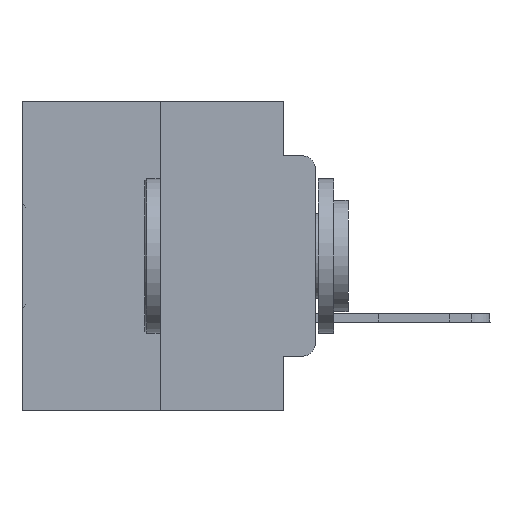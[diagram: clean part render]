
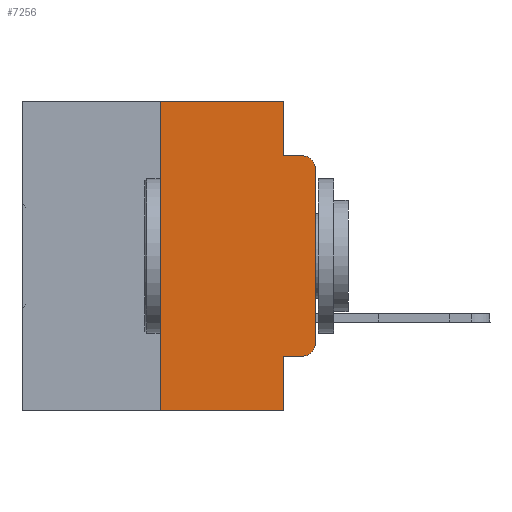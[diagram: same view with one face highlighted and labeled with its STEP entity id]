
A CAD part, left-side view. The second image highlights one B-rep face of the part: STEP entity #7256.
In plain terms, the highlighted planar face has unit normal (-1, 0, 0).
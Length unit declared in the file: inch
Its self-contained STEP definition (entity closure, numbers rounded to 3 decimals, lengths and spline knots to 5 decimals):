
#453 = DIRECTION ( 'NONE',  ( 0., -1., 0. ) ) ;
#516 = VECTOR ( 'NONE', #11268, 39.37008 ) ;
#835 = VECTOR ( 'NONE', #15835, 39.37008 ) ;
#908 = CARTESIAN_POINT ( 'NONE',  ( 0., 0., -0.1085 ) ) ;
#976 = ORIENTED_EDGE ( 'NONE', *, *, #17083, .F. ) ;
#977 = EDGE_CURVE ( 'NONE', #14115, #31015, #20515, .T. ) ;
#1703 = CARTESIAN_POINT ( 'NONE',  ( 0., 0.051, -0.5 ) ) ;
#2114 = DIRECTION ( 'NONE',  ( 0., 0., -1. ) ) ;
#2236 = DIRECTION ( 'NONE',  ( 0., 0., -1. ) ) ;
#2486 = VECTOR ( 'NONE', #23455, 39.37008 ) ;
#2603 = CARTESIAN_POINT ( 'NONE',  ( 0., 0.051, -0.4115 ) ) ;
#2642 = VECTOR ( 'NONE', #12269, 39.37008 ) ;
#3105 = LINE ( 'NONE', #22414, #14144 ) ;
#3440 = ORIENTED_EDGE ( 'NONE', *, *, #977, .T. ) ;
#3738 = CARTESIAN_POINT ( 'NONE',  ( 0., 0.473, -0.5 ) ) ;
#3914 = EDGE_CURVE ( 'NONE', #7115, #31190, #22333, .T. ) ;
#4561 = CARTESIAN_POINT ( 'NONE',  ( 0., 0.051, -0.4115 ) ) ;
#4764 = ORIENTED_EDGE ( 'NONE', *, *, #13212, .F. ) ;
#5065 = AXIS2_PLACEMENT_3D ( 'NONE', #32274, #27254, #2236 ) ;
#5093 = ORIENTED_EDGE ( 'NONE', *, *, #24592, .T. ) ;
#5542 = AXIS2_PLACEMENT_3D ( 'NONE', #16052, #14402, #2114 ) ;
#5765 = LINE ( 'NONE', #27186, #2642 ) ;
#6087 = LINE ( 'NONE', #6248, #516 ) ;
#6248 = CARTESIAN_POINT ( 'NONE',  ( 0., 0.051, 0. ) ) ;
#6380 = VECTOR ( 'NONE', #22400, 39.37008 ) ;
#6598 = VERTEX_POINT ( 'NONE', #2603 ) ;
#7115 = VERTEX_POINT ( 'NONE', #9349 ) ;
#7256 = ADVANCED_FACE ( 'NONE', ( #15654 ), #22505, .F. ) ;
#7352 = CARTESIAN_POINT ( 'NONE',  ( 0., 0.25, 0. ) ) ;
#7557 = LINE ( 'NONE', #13187, #835 ) ;
#8166 = ORIENTED_EDGE ( 'NONE', *, *, #15887, .F. ) ;
#9242 = VERTEX_POINT ( 'NONE', #18804 ) ;
#9349 = CARTESIAN_POINT ( 'NONE',  ( 0., 0.02, -0.4115 ) ) ;
#9386 = ORIENTED_EDGE ( 'NONE', *, *, #14272, .F. ) ;
#10572 = LINE ( 'NONE', #18261, #20709 ) ;
#11268 = DIRECTION ( 'NONE',  ( 0., 0., -1. ) ) ;
#12269 = DIRECTION ( 'NONE',  ( 0., 0., 1. ) ) ;
#13023 = LINE ( 'NONE', #4561, #6380 ) ;
#13187 = CARTESIAN_POINT ( 'NONE',  ( 0., 0.051, 0. ) ) ;
#13212 = EDGE_CURVE ( 'NONE', #9242, #22524, #6087, .T. ) ;
#14115 = VERTEX_POINT ( 'NONE', #19571 ) ;
#14144 = VECTOR ( 'NONE', #17814, 39.37008 ) ;
#14272 = EDGE_CURVE ( 'NONE', #6598, #31015, #7557, .T. ) ;
#14347 = ORIENTED_EDGE ( 'NONE', *, *, #29134, .T. ) ;
#14402 = DIRECTION ( 'NONE',  ( -1., 0., 0. ) ) ;
#15159 = AXIS2_PLACEMENT_3D ( 'NONE', #26997, #21621, #26676 ) ;
#15654 = FACE_OUTER_BOUND ( 'NONE', #16497, .T. ) ;
#15835 = DIRECTION ( 'NONE',  ( 0., 0., -1. ) ) ;
#15887 = EDGE_CURVE ( 'NONE', #22524, #17123, #10572, .T. ) ;
#16052 = CARTESIAN_POINT ( 'NONE',  ( 0., 0.02, -0.3915 ) ) ;
#16083 = CARTESIAN_POINT ( 'NONE',  ( 0., 0.473, 0. ) ) ;
#16219 = CARTESIAN_POINT ( 'NONE',  ( 0., 0.051, -0.0885 ) ) ;
#16497 = EDGE_LOOP ( 'NONE', ( #14347, #32001, #8166, #4764, #19556, #976, #3440, #9386, #5093, #29952 ) ) ;
#17083 = EDGE_CURVE ( 'NONE', #14115, #22117, #5765, .T. ) ;
#17123 = VERTEX_POINT ( 'NONE', #30066 ) ;
#17158 = EDGE_CURVE ( 'NONE', #22117, #9242, #25778, .T. ) ;
#17814 = DIRECTION ( 'NONE',  ( 0., 0., 1. ) ) ;
#18261 = CARTESIAN_POINT ( 'NONE',  ( 0., 0.051, -0.0885 ) ) ;
#18804 = CARTESIAN_POINT ( 'NONE',  ( 0., 0.051, 0. ) ) ;
#19556 = ORIENTED_EDGE ( 'NONE', *, *, #17158, .F. ) ;
#19571 = CARTESIAN_POINT ( 'NONE',  ( 0., 0.25, -0.5 ) ) ;
#20515 = LINE ( 'NONE', #3738, #2486 ) ;
#20709 = VECTOR ( 'NONE', #453, 39.37008 ) ;
#21303 = CIRCLE ( 'NONE', #15159, 0.02 ) ;
#21621 = DIRECTION ( 'NONE',  ( -1., 0., 0. ) ) ;
#22117 = VERTEX_POINT ( 'NONE', #7352 ) ;
#22333 = CIRCLE ( 'NONE', #5542, 0.02 ) ;
#22400 = DIRECTION ( 'NONE',  ( 0., -1., 0. ) ) ;
#22414 = CARTESIAN_POINT ( 'NONE',  ( 0., 0., 0. ) ) ;
#22505 = PLANE ( 'NONE',  #5065 ) ;
#22524 = VERTEX_POINT ( 'NONE', #16219 ) ;
#22960 = VERTEX_POINT ( 'NONE', #908 ) ;
#23161 = DIRECTION ( 'NONE',  ( 0., -1., 0. ) ) ;
#23455 = DIRECTION ( 'NONE',  ( 0., -1., 0. ) ) ;
#24592 = EDGE_CURVE ( 'NONE', #6598, #7115, #13023, .T. ) ;
#25778 = LINE ( 'NONE', #16083, #27001 ) ;
#26676 = DIRECTION ( 'NONE',  ( 0., 0., -1. ) ) ;
#26838 = EDGE_CURVE ( 'NONE', #22960, #17123, #21303, .T. ) ;
#26997 = CARTESIAN_POINT ( 'NONE',  ( 0., 0.02, -0.1085 ) ) ;
#27001 = VECTOR ( 'NONE', #23161, 39.37008 ) ;
#27186 = CARTESIAN_POINT ( 'NONE',  ( 0., 0.25, 0. ) ) ;
#27254 = DIRECTION ( 'NONE',  ( 1., 0., 0. ) ) ;
#27657 = CARTESIAN_POINT ( 'NONE',  ( 0., 0., -0.3915 ) ) ;
#29134 = EDGE_CURVE ( 'NONE', #31190, #22960, #3105, .T. ) ;
#29952 = ORIENTED_EDGE ( 'NONE', *, *, #3914, .T. ) ;
#30066 = CARTESIAN_POINT ( 'NONE',  ( 0., 0.02, -0.0885 ) ) ;
#31015 = VERTEX_POINT ( 'NONE', #1703 ) ;
#31190 = VERTEX_POINT ( 'NONE', #27657 ) ;
#32001 = ORIENTED_EDGE ( 'NONE', *, *, #26838, .T. ) ;
#32274 = CARTESIAN_POINT ( 'NONE',  ( 0., 0.473, 0. ) ) ;
